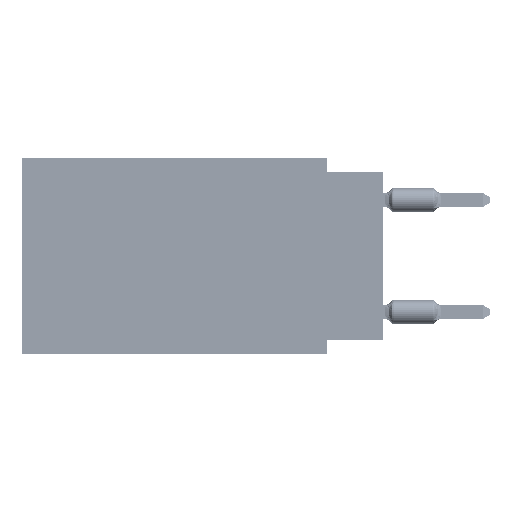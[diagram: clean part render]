
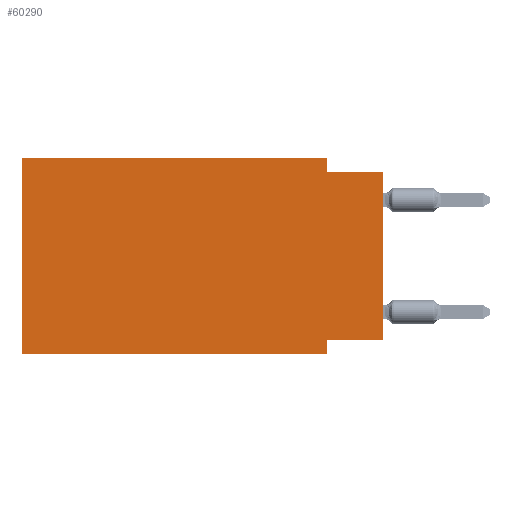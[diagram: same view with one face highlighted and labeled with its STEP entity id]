
A CAD part, left-side view. The second image highlights one B-rep face of the part: STEP entity #60290.
In plain terms, the highlighted planar face has unit normal (-1, 0, 0).
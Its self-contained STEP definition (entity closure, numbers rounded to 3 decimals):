
#96 = VERTEX_POINT ( 'NONE', #75801 ) ;
#1130 = VECTOR ( 'NONE', #109887, 1000. ) ;
#1529 = VERTEX_POINT ( 'NONE', #61908 ) ;
#2076 = AXIS2_PLACEMENT_3D ( 'NONE', #3281, #39042, #38471 ) ;
#2083 = CARTESIAN_POINT ( 'NONE',  ( 0., 2.54, -8.255 ) ) ;
#3281 = CARTESIAN_POINT ( 'NONE',  ( 0., 16.383, 0. ) ) ;
#9961 = CARTESIAN_POINT ( 'NONE',  ( 0., 16.383, 0. ) ) ;
#10883 = ORIENTED_EDGE ( 'NONE', *, *, #71368, .T. ) ;
#12885 = VERTEX_POINT ( 'NONE', #80214 ) ;
#13022 = VECTOR ( 'NONE', #75626, 1000. ) ;
#16468 = CARTESIAN_POINT ( 'NONE',  ( 0., 0., -0.635 ) ) ;
#17473 = ORIENTED_EDGE ( 'NONE', *, *, #86509, .F. ) ;
#18580 = EDGE_CURVE ( 'NONE', #62545, #26871, #22825, .T. ) ;
#21823 = CARTESIAN_POINT ( 'NONE',  ( 0., 2.54, -8.89 ) ) ;
#22825 = LINE ( 'NONE', #58537, #1130 ) ;
#25221 = EDGE_LOOP ( 'NONE', ( #10883, #52746, #47713, #62390, #90920, #63176, #17473, #26957 ) ) ;
#26720 = CARTESIAN_POINT ( 'NONE',  ( 0., 2.54, 0. ) ) ;
#26871 = VERTEX_POINT ( 'NONE', #77670 ) ;
#26957 = ORIENTED_EDGE ( 'NONE', *, *, #105856, .F. ) ;
#27394 = DIRECTION ( 'NONE',  ( 0., -1., 0. ) ) ;
#31965 = CARTESIAN_POINT ( 'NONE',  ( 0., 0., 0. ) ) ;
#33028 = VECTOR ( 'NONE', #82811, 1000. ) ;
#38471 = DIRECTION ( 'NONE',  ( 0., 0., -1. ) ) ;
#39042 = DIRECTION ( 'NONE',  ( 1., 0., 0. ) ) ;
#45124 = DIRECTION ( 'NONE',  ( 0., -1., 0. ) ) ;
#46212 = VECTOR ( 'NONE', #45124, 1000. ) ;
#46479 = LINE ( 'NONE', #72462, #33028 ) ;
#47713 = ORIENTED_EDGE ( 'NONE', *, *, #18580, .F. ) ;
#51478 = DIRECTION ( 'NONE',  ( 0., 0., 1. ) ) ;
#52130 = VECTOR ( 'NONE', #27394, 1000. ) ;
#52277 = EDGE_CURVE ( 'NONE', #26871, #12885, #52777, .T. ) ;
#52746 = ORIENTED_EDGE ( 'NONE', *, *, #52277, .F. ) ;
#52777 = LINE ( 'NONE', #16468, #52130 ) ;
#56466 = EDGE_CURVE ( 'NONE', #1529, #96, #110936, .T. ) ;
#57276 = DIRECTION ( 'NONE',  ( 0., 0., 1. ) ) ;
#58134 = EDGE_CURVE ( 'NONE', #1529, #98691, #92948, .T. ) ;
#58537 = CARTESIAN_POINT ( 'NONE',  ( 0., 2.54, 0. ) ) ;
#60290 = ADVANCED_FACE ( 'NONE', ( #107125 ), #108250, .F. ) ;
#61908 = CARTESIAN_POINT ( 'NONE',  ( 0., 16.383, -8.89 ) ) ;
#62390 = ORIENTED_EDGE ( 'NONE', *, *, #65760, .F. ) ;
#62545 = VERTEX_POINT ( 'NONE', #26720 ) ;
#63176 = ORIENTED_EDGE ( 'NONE', *, *, #58134, .T. ) ;
#63905 = CARTESIAN_POINT ( 'NONE',  ( 0., 0., -8.255 ) ) ;
#65760 = EDGE_CURVE ( 'NONE', #96, #62545, #69943, .T. ) ;
#69587 = VECTOR ( 'NONE', #57276, 1000. ) ;
#69943 = LINE ( 'NONE', #9961, #46212 ) ;
#71368 = EDGE_CURVE ( 'NONE', #104223, #12885, #94196, .T. ) ;
#72462 = CARTESIAN_POINT ( 'NONE',  ( 0., 0., -8.255 ) ) ;
#74599 = CARTESIAN_POINT ( 'NONE',  ( 0., 16.383, 0. ) ) ;
#75195 = VERTEX_POINT ( 'NONE', #2083 ) ;
#75626 = DIRECTION ( 'NONE',  ( 0., -1., 0. ) ) ;
#75801 = CARTESIAN_POINT ( 'NONE',  ( 0., 16.383, 0. ) ) ;
#77670 = CARTESIAN_POINT ( 'NONE',  ( 0., 2.54, -0.635 ) ) ;
#80214 = CARTESIAN_POINT ( 'NONE',  ( 0., 0., -0.635 ) ) ;
#82811 = DIRECTION ( 'NONE',  ( 0., 1., 0. ) ) ;
#86509 = EDGE_CURVE ( 'NONE', #75195, #98691, #103555, .T. ) ;
#90920 = ORIENTED_EDGE ( 'NONE', *, *, #56466, .F. ) ;
#92948 = LINE ( 'NONE', #93497, #13022 ) ;
#93497 = CARTESIAN_POINT ( 'NONE',  ( 0., 16.383, -8.89 ) ) ;
#94196 = LINE ( 'NONE', #31965, #103413 ) ;
#94324 = DIRECTION ( 'NONE',  ( 0., 0., -1. ) ) ;
#95520 = VECTOR ( 'NONE', #94324, 1000. ) ;
#98691 = VERTEX_POINT ( 'NONE', #21823 ) ;
#103413 = VECTOR ( 'NONE', #51478, 1000. ) ;
#103555 = LINE ( 'NONE', #112201, #95520 ) ;
#104223 = VERTEX_POINT ( 'NONE', #63905 ) ;
#105856 = EDGE_CURVE ( 'NONE', #104223, #75195, #46479, .T. ) ;
#107125 = FACE_OUTER_BOUND ( 'NONE', #25221, .T. ) ;
#108250 = PLANE ( 'NONE',  #2076 ) ;
#109887 = DIRECTION ( 'NONE',  ( 0., 0., -1. ) ) ;
#110936 = LINE ( 'NONE', #74599, #69587 ) ;
#112201 = CARTESIAN_POINT ( 'NONE',  ( 0., 2.54, -8.89 ) ) ;
